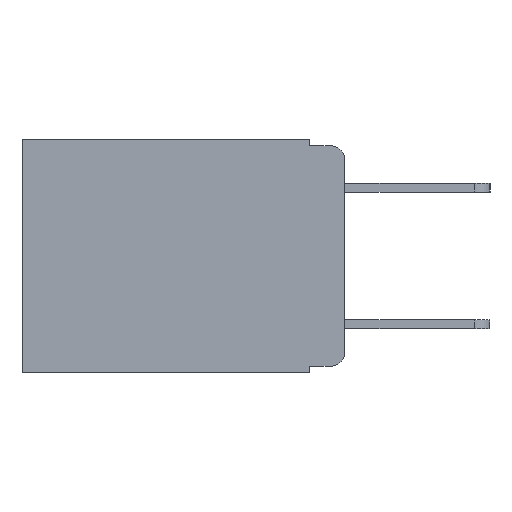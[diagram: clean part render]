
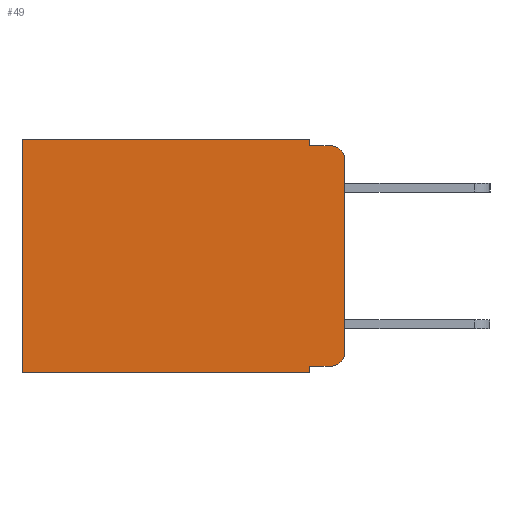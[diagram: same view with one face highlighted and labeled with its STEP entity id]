
A CAD part, left-side view. The second image highlights one B-rep face of the part: STEP entity #49.
In plain terms, the highlighted planar face has unit normal (-1, 0, 0).
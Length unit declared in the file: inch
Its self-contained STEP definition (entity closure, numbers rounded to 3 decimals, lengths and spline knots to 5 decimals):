
#49 = ADVANCED_FACE ( 'NONE', ( #3623 ), #7601, .F. ) ;
#552 = CARTESIAN_POINT ( 'NONE',  ( 0.298, 0., 0. ) ) ;
#736 = CARTESIAN_POINT ( 'NONE',  ( 0.298, 0.02, -0.313 ) ) ;
#748 = EDGE_CURVE ( 'NONE', #16397, #4777, #1041, .T. ) ;
#902 = VERTEX_POINT ( 'NONE', #13124 ) ;
#911 = LINE ( 'NONE', #10544, #8785 ) ;
#1041 = LINE ( 'NONE', #16818, #8197 ) ;
#1101 = VERTEX_POINT ( 'NONE', #9844 ) ;
#1198 = DIRECTION ( 'NONE',  ( 0., 0., -1. ) ) ;
#1348 = AXIS2_PLACEMENT_3D ( 'NONE', #16176, #13972, #13954 ) ;
#1417 = ORIENTED_EDGE ( 'NONE', *, *, #11433, .T. ) ;
#1882 = VECTOR ( 'NONE', #1968, 39.37008 ) ;
#1938 = LINE ( 'NONE', #3567, #16411 ) ;
#1968 = DIRECTION ( 'NONE',  ( 0., -1., 0. ) ) ;
#2358 = CARTESIAN_POINT ( 'NONE',  ( 0.298, 0., -0.03 ) ) ;
#2371 = DIRECTION ( 'NONE',  ( 0., 0., -1. ) ) ;
#2612 = VERTEX_POINT ( 'NONE', #17812 ) ;
#2770 = DIRECTION ( 'NONE',  ( 0., 1., 0. ) ) ;
#3279 = DIRECTION ( 'NONE',  ( 0., 1., 0. ) ) ;
#3404 = CARTESIAN_POINT ( 'NONE',  ( 0.298, 0., 0. ) ) ;
#3567 = CARTESIAN_POINT ( 'NONE',  ( 0.298, 0., -0.343 ) ) ;
#3623 = FACE_OUTER_BOUND ( 'NONE', #6687, .T. ) ;
#3975 = EDGE_CURVE ( 'NONE', #8312, #12522, #5642, .T. ) ;
#3997 = VERTEX_POINT ( 'NONE', #15840 ) ;
#4091 = AXIS2_PLACEMENT_3D ( 'NONE', #552, #11931, #1198 ) ;
#4639 = VECTOR ( 'NONE', #18011, 39.37008 ) ;
#4777 = VERTEX_POINT ( 'NONE', #8823 ) ;
#4849 = DIRECTION ( 'NONE',  ( 0., 0., -1. ) ) ;
#4985 = EDGE_CURVE ( 'NONE', #14462, #9722, #6725, .T. ) ;
#5343 = EDGE_CURVE ( 'NONE', #3997, #1101, #11940, .T. ) ;
#5642 = CIRCLE ( 'NONE', #1348, 0.02 ) ;
#5923 = LINE ( 'NONE', #17655, #1882 ) ;
#6305 = EDGE_CURVE ( 'NONE', #9722, #1101, #1938, .T. ) ;
#6687 = EDGE_LOOP ( 'NONE', ( #10791, #10125, #7846, #16599, #17604, #16731, #15982, #18093, #13698, #1417 ) ) ;
#6725 = LINE ( 'NONE', #14219, #17032 ) ;
#7053 = DIRECTION ( 'NONE',  ( 0., -1., 0. ) ) ;
#7100 = EDGE_CURVE ( 'NONE', #16397, #3997, #10295, .T. ) ;
#7573 = EDGE_CURVE ( 'NONE', #14462, #2612, #5923, .T. ) ;
#7601 = PLANE ( 'NONE',  #4091 ) ;
#7846 = ORIENTED_EDGE ( 'NONE', *, *, #15831, .F. ) ;
#8197 = VECTOR ( 'NONE', #4849, 39.37008 ) ;
#8312 = VERTEX_POINT ( 'NONE', #2358 ) ;
#8785 = VECTOR ( 'NONE', #13426, 39.37008 ) ;
#8818 = LINE ( 'NONE', #12802, #12249 ) ;
#8823 = CARTESIAN_POINT ( 'NONE',  ( 0.298, 0.051, -0.01 ) ) ;
#9115 = CIRCLE ( 'NONE', #12780, 0.02 ) ;
#9530 = CARTESIAN_POINT ( 'NONE',  ( 0.298, 0.051, -0.333 ) ) ;
#9722 = VERTEX_POINT ( 'NONE', #17085 ) ;
#9844 = CARTESIAN_POINT ( 'NONE',  ( 0.298, 0.473, -0.343 ) ) ;
#10125 = ORIENTED_EDGE ( 'NONE', *, *, #3975, .T. ) ;
#10295 = LINE ( 'NONE', #3404, #17964 ) ;
#10544 = CARTESIAN_POINT ( 'NONE',  ( 0.298, 0., 0. ) ) ;
#10791 = ORIENTED_EDGE ( 'NONE', *, *, #18234, .F. ) ;
#11246 = DIRECTION ( 'NONE',  ( -1., 0., 0. ) ) ;
#11433 = EDGE_CURVE ( 'NONE', #2612, #902, #9115, .T. ) ;
#11931 = DIRECTION ( 'NONE',  ( 1., 0., 0. ) ) ;
#11940 = LINE ( 'NONE', #12346, #4639 ) ;
#12249 = VECTOR ( 'NONE', #7053, 39.37008 ) ;
#12346 = CARTESIAN_POINT ( 'NONE',  ( 0.298, 0.473, 0. ) ) ;
#12522 = VERTEX_POINT ( 'NONE', #17560 ) ;
#12780 = AXIS2_PLACEMENT_3D ( 'NONE', #736, #11246, #2371 ) ;
#12802 = CARTESIAN_POINT ( 'NONE',  ( 0.298, 0.051, -0.01 ) ) ;
#12816 = DIRECTION ( 'NONE',  ( 0., 0., -1. ) ) ;
#13124 = CARTESIAN_POINT ( 'NONE',  ( 0.298, 0., -0.313 ) ) ;
#13426 = DIRECTION ( 'NONE',  ( 0., 0., -1. ) ) ;
#13698 = ORIENTED_EDGE ( 'NONE', *, *, #7573, .T. ) ;
#13954 = DIRECTION ( 'NONE',  ( 0., 0., -1. ) ) ;
#13972 = DIRECTION ( 'NONE',  ( -1., 0., 0. ) ) ;
#14219 = CARTESIAN_POINT ( 'NONE',  ( 0.298, 0.051, 0. ) ) ;
#14462 = VERTEX_POINT ( 'NONE', #9530 ) ;
#15831 = EDGE_CURVE ( 'NONE', #4777, #12522, #8818, .T. ) ;
#15840 = CARTESIAN_POINT ( 'NONE',  ( 0.298, 0.473, 0. ) ) ;
#15982 = ORIENTED_EDGE ( 'NONE', *, *, #6305, .F. ) ;
#16176 = CARTESIAN_POINT ( 'NONE',  ( 0.298, 0.02, -0.03 ) ) ;
#16397 = VERTEX_POINT ( 'NONE', #17705 ) ;
#16411 = VECTOR ( 'NONE', #2770, 39.37008 ) ;
#16599 = ORIENTED_EDGE ( 'NONE', *, *, #748, .F. ) ;
#16731 = ORIENTED_EDGE ( 'NONE', *, *, #5343, .T. ) ;
#16818 = CARTESIAN_POINT ( 'NONE',  ( 0.298, 0.051, 0. ) ) ;
#17032 = VECTOR ( 'NONE', #12816, 39.37008 ) ;
#17085 = CARTESIAN_POINT ( 'NONE',  ( 0.298, 0.051, -0.343 ) ) ;
#17560 = CARTESIAN_POINT ( 'NONE',  ( 0.298, 0.02, -0.01 ) ) ;
#17604 = ORIENTED_EDGE ( 'NONE', *, *, #7100, .T. ) ;
#17655 = CARTESIAN_POINT ( 'NONE',  ( 0.298, 0.051, -0.333 ) ) ;
#17705 = CARTESIAN_POINT ( 'NONE',  ( 0.298, 0.051, 0. ) ) ;
#17812 = CARTESIAN_POINT ( 'NONE',  ( 0.298, 0.02, -0.333 ) ) ;
#17964 = VECTOR ( 'NONE', #3279, 39.37008 ) ;
#18011 = DIRECTION ( 'NONE',  ( 0., 0., -1. ) ) ;
#18093 = ORIENTED_EDGE ( 'NONE', *, *, #4985, .F. ) ;
#18234 = EDGE_CURVE ( 'NONE', #8312, #902, #911, .T. ) ;
